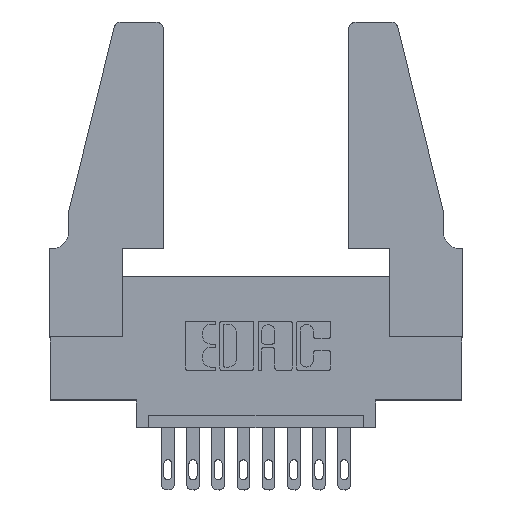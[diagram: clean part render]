
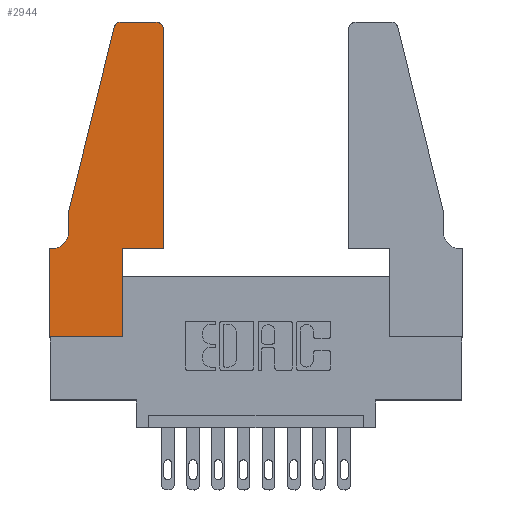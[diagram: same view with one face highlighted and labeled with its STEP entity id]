
A CAD part, top view. The second image highlights one B-rep face of the part: STEP entity #2944.
In plain terms, the highlighted planar face has unit normal (0, 0, 1).
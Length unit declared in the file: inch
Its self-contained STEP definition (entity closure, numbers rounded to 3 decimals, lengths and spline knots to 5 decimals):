
#177 = LINE ( 'NONE', #8033, #10572 ) ;
#257 = CARTESIAN_POINT ( 'NONE',  ( 0.4505, 0.35, 0.37 ) ) ;
#307 = EDGE_CURVE ( 'NONE', #5839, #2707, #10604, .T. ) ;
#438 = AXIS2_PLACEMENT_3D ( 'NONE', #692, #5936, #7902 ) ;
#443 = CARTESIAN_POINT ( 'NONE',  ( 0., 0., 0.37 ) ) ;
#692 = CARTESIAN_POINT ( 'NONE',  ( 0.0055, 0.42, 0.37 ) ) ;
#733 = VERTEX_POINT ( 'NONE', #8167 ) ;
#772 = CARTESIAN_POINT ( 'NONE',  ( 0.4505, 0.35, 0.37 ) ) ;
#984 = CIRCLE ( 'NONE', #4233, 0.03 ) ;
#1223 = EDGE_CURVE ( 'NONE', #3813, #5839, #177, .T. ) ;
#1305 = CARTESIAN_POINT ( 'NONE',  ( 0.4505, 0.35, 0.37 ) ) ;
#1510 = CARTESIAN_POINT ( 'NONE',  ( 0.284, 1.25, 0.37 ) ) ;
#1732 = ORIENTED_EDGE ( 'NONE', *, *, #3680, .T. ) ;
#2242 = CIRCLE ( 'NONE', #438, 0.07 ) ;
#2344 = EDGE_CURVE ( 'NONE', #4668, #3813, #11153, .T. ) ;
#2362 = EDGE_CURVE ( 'NONE', #11621, #733, #4479, .T. ) ;
#2707 = VERTEX_POINT ( 'NONE', #3407 ) ;
#2930 = LINE ( 'NONE', #257, #9143 ) ;
#2944 = ADVANCED_FACE ( 'NONE', ( #4934 ), #3873, .T. ) ;
#3080 = VECTOR ( 'NONE', #3405, 39.37008 ) ;
#3120 = DIRECTION ( 'NONE',  ( 0., 1., 0. ) ) ;
#3248 = EDGE_CURVE ( 'NONE', #2707, #11431, #9777, .T. ) ;
#3250 = DIRECTION ( 'NONE',  ( 0., 1., 0. ) ) ;
#3310 = EDGE_CURVE ( 'NONE', #9460, #11467, #2930, .T. ) ;
#3405 = DIRECTION ( 'NONE',  ( -0.239, -0.971, 0. ) ) ;
#3407 = CARTESIAN_POINT ( 'NONE',  ( 0.2865, 0., 0.37 ) ) ;
#3680 = EDGE_CURVE ( 'NONE', #11485, #11621, #6794, .T. ) ;
#3701 = DIRECTION ( 'NONE',  ( -1., 0., 0. ) ) ;
#3764 = ORIENTED_EDGE ( 'NONE', *, *, #8533, .T. ) ;
#3813 = VERTEX_POINT ( 'NONE', #5150 ) ;
#3820 = LINE ( 'NONE', #10477, #6631 ) ;
#3873 = PLANE ( 'NONE',  #8243 ) ;
#3932 = ORIENTED_EDGE ( 'NONE', *, *, #8458, .T. ) ;
#4096 = DIRECTION ( 'NONE',  ( 0., -1., 0. ) ) ;
#4225 = EDGE_CURVE ( 'NONE', #11431, #9460, #5843, .T. ) ;
#4233 = AXIS2_PLACEMENT_3D ( 'NONE', #5374, #8381, #5471 ) ;
#4479 = LINE ( 'NONE', #9846, #5116 ) ;
#4590 = DIRECTION ( 'NONE',  ( 1., 0., 0. ) ) ;
#4668 = VERTEX_POINT ( 'NONE', #8469 ) ;
#4672 = ORIENTED_EDGE ( 'NONE', *, *, #307, .T. ) ;
#4796 = CARTESIAN_POINT ( 'NONE',  ( 0.2865, 0.35, 0.37 ) ) ;
#4934 = FACE_OUTER_BOUND ( 'NONE', #8029, .T. ) ;
#5116 = VECTOR ( 'NONE', #9889, 39.37008 ) ;
#5150 = CARTESIAN_POINT ( 'NONE',  ( 0., 0.35, 0.37 ) ) ;
#5374 = CARTESIAN_POINT ( 'NONE',  ( 0.284, 1.22, 0.37 ) ) ;
#5446 = ORIENTED_EDGE ( 'NONE', *, *, #4225, .T. ) ;
#5471 = DIRECTION ( 'NONE',  ( 1., 0., 0. ) ) ;
#5697 = CARTESIAN_POINT ( 'NONE',  ( 0., 0.35, 0.37 ) ) ;
#5730 = CIRCLE ( 'NONE', #7810, 0.03 ) ;
#5839 = VERTEX_POINT ( 'NONE', #443 ) ;
#5843 = LINE ( 'NONE', #1305, #10807 ) ;
#5936 = DIRECTION ( 'NONE',  ( 0., 0., -1. ) ) ;
#6078 = CARTESIAN_POINT ( 'NONE',  ( 0.4205, 1.22, 0.37 ) ) ;
#6182 = CARTESIAN_POINT ( 'NONE',  ( 0.2865, 0.35, 0.37 ) ) ;
#6262 = VERTEX_POINT ( 'NONE', #10320 ) ;
#6539 = VECTOR ( 'NONE', #11089, 39.37008 ) ;
#6631 = VECTOR ( 'NONE', #3701, 39.37008 ) ;
#6794 = LINE ( 'NONE', #9436, #3080 ) ;
#6853 = CARTESIAN_POINT ( 'NONE',  ( 0.4505, 1.22, 0.37 ) ) ;
#6952 = DIRECTION ( 'NONE',  ( 0., 0., 1. ) ) ;
#7112 = EDGE_CURVE ( 'NONE', #6262, #7994, #3820, .T. ) ;
#7359 = VECTOR ( 'NONE', #4590, 39.37008 ) ;
#7735 = CARTESIAN_POINT ( 'NONE',  ( 0.0755, 0.5, 0.37 ) ) ;
#7810 = AXIS2_PLACEMENT_3D ( 'NONE', #6078, #6952, #8008 ) ;
#7902 = DIRECTION ( 'NONE',  ( -1., 0., 0. ) ) ;
#7994 = VERTEX_POINT ( 'NONE', #1510 ) ;
#8008 = DIRECTION ( 'NONE',  ( 1., 0., 0. ) ) ;
#8029 = EDGE_LOOP ( 'NONE', ( #10131, #3932, #1732, #12753, #3764, #9997, #9696, #4672, #10436, #5446, #10985, #8614 ) ) ;
#8033 = CARTESIAN_POINT ( 'NONE',  ( 0., 0., 0.37 ) ) ;
#8167 = CARTESIAN_POINT ( 'NONE',  ( 0.0755, 0.42, 0.37 ) ) ;
#8243 = AXIS2_PLACEMENT_3D ( 'NONE', #5697, #12670, #12625 ) ;
#8381 = DIRECTION ( 'NONE',  ( 0., 0., 1. ) ) ;
#8458 = EDGE_CURVE ( 'NONE', #7994, #11485, #984, .T. ) ;
#8469 = CARTESIAN_POINT ( 'NONE',  ( 0.0055, 0.35, 0.37 ) ) ;
#8533 = EDGE_CURVE ( 'NONE', #733, #4668, #2242, .T. ) ;
#8614 = ORIENTED_EDGE ( 'NONE', *, *, #11022, .T. ) ;
#9143 = VECTOR ( 'NONE', #3250, 39.37008 ) ;
#9436 = CARTESIAN_POINT ( 'NONE',  ( 0.0755, 0.5, 0.37 ) ) ;
#9460 = VERTEX_POINT ( 'NONE', #772 ) ;
#9696 = ORIENTED_EDGE ( 'NONE', *, *, #1223, .T. ) ;
#9777 = LINE ( 'NONE', #6182, #12389 ) ;
#9846 = CARTESIAN_POINT ( 'NONE',  ( 0.0755, 0.5, 0.37 ) ) ;
#9889 = DIRECTION ( 'NONE',  ( 0., -1., 0. ) ) ;
#9935 = CARTESIAN_POINT ( 'NONE',  ( 0.25487, 1.22718, 0.37 ) ) ;
#9997 = ORIENTED_EDGE ( 'NONE', *, *, #2344, .T. ) ;
#10061 = CARTESIAN_POINT ( 'NONE',  ( 0.0755, 0.35, 0.37 ) ) ;
#10131 = ORIENTED_EDGE ( 'NONE', *, *, #7112, .T. ) ;
#10320 = CARTESIAN_POINT ( 'NONE',  ( 0.4205, 1.25, 0.37 ) ) ;
#10436 = ORIENTED_EDGE ( 'NONE', *, *, #3248, .T. ) ;
#10477 = CARTESIAN_POINT ( 'NONE',  ( 0.2605, 1.25, 0.37 ) ) ;
#10572 = VECTOR ( 'NONE', #4096, 39.37008 ) ;
#10604 = LINE ( 'NONE', #12568, #7359 ) ;
#10807 = VECTOR ( 'NONE', #12299, 39.37008 ) ;
#10985 = ORIENTED_EDGE ( 'NONE', *, *, #3310, .T. ) ;
#11022 = EDGE_CURVE ( 'NONE', #11467, #6262, #5730, .T. ) ;
#11089 = DIRECTION ( 'NONE',  ( -1., 0., 0. ) ) ;
#11153 = LINE ( 'NONE', #10061, #6539 ) ;
#11431 = VERTEX_POINT ( 'NONE', #4796 ) ;
#11467 = VERTEX_POINT ( 'NONE', #6853 ) ;
#11485 = VERTEX_POINT ( 'NONE', #9935 ) ;
#11621 = VERTEX_POINT ( 'NONE', #7735 ) ;
#12299 = DIRECTION ( 'NONE',  ( 1., 0., 0. ) ) ;
#12389 = VECTOR ( 'NONE', #3120, 39.37008 ) ;
#12568 = CARTESIAN_POINT ( 'NONE',  ( 0., 0., 0.37 ) ) ;
#12625 = DIRECTION ( 'NONE',  ( 1., 0., 0. ) ) ;
#12670 = DIRECTION ( 'NONE',  ( 0., 0., 1. ) ) ;
#12753 = ORIENTED_EDGE ( 'NONE', *, *, #2362, .T. ) ;
